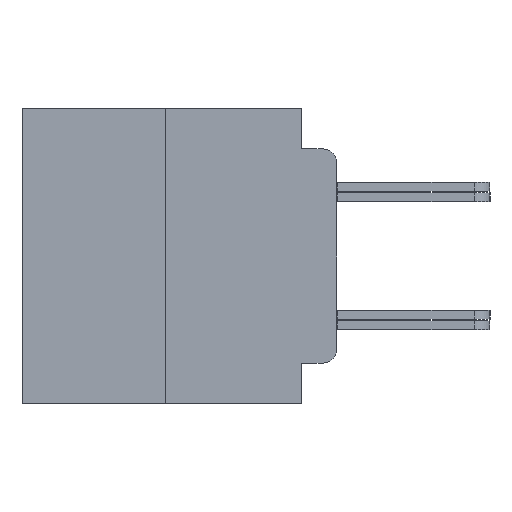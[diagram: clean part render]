
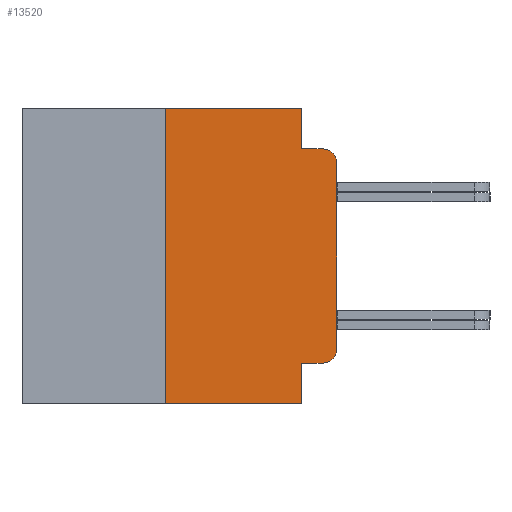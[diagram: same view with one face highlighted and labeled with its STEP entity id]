
A CAD part, left-side view. The second image highlights one B-rep face of the part: STEP entity #13520.
In plain terms, the highlighted planar face has unit normal (-1, 0, 0).
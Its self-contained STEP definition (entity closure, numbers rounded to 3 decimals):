
#203 = CARTESIAN_POINT ( 'NONE',  ( -75.603, 0.508, -3.975 ) ) ;
#330 = VECTOR ( 'NONE', #15667, 1000. ) ;
#479 = VERTEX_POINT ( 'NONE', #25853 ) ;
#786 = CARTESIAN_POINT ( 'NONE',  ( -75.603, 0.508, 3.467 ) ) ;
#1396 = LINE ( 'NONE', #4190, #27976 ) ;
#1812 = LINE ( 'NONE', #8970, #3211 ) ;
#2841 = CARTESIAN_POINT ( 'NONE',  ( -75.603, 0., -3.467 ) ) ;
#2872 = EDGE_CURVE ( 'NONE', #10562, #11289, #6207, .T. ) ;
#2905 = EDGE_CURVE ( 'NONE', #21259, #26325, #23056, .T. ) ;
#3078 = CARTESIAN_POINT ( 'NONE',  ( -75.603, 11.684, 5.486 ) ) ;
#3211 = VECTOR ( 'NONE', #4315, 1000. ) ;
#3571 = ORIENTED_EDGE ( 'NONE', *, *, #21143, .T. ) ;
#3697 = CARTESIAN_POINT ( 'NONE',  ( -75.603, 1.295, 0. ) ) ;
#3964 = VERTEX_POINT ( 'NONE', #2841 ) ;
#4078 = LINE ( 'NONE', #3697, #5091 ) ;
#4190 = CARTESIAN_POINT ( 'NONE',  ( -75.603, 0., 5.486 ) ) ;
#4315 = DIRECTION ( 'NONE',  ( 0., -1., 0. ) ) ;
#4521 = EDGE_CURVE ( 'NONE', #21259, #25367, #4078, .T. ) ;
#4785 = ORIENTED_EDGE ( 'NONE', *, *, #12134, .F. ) ;
#4992 = DIRECTION ( 'NONE',  ( 1., 0., 0. ) ) ;
#5076 = ORIENTED_EDGE ( 'NONE', *, *, #2905, .T. ) ;
#5091 = VECTOR ( 'NONE', #10548, 1000. ) ;
#5511 = DIRECTION ( 'NONE',  ( -1., 0., 0. ) ) ;
#6097 = CIRCLE ( 'NONE', #24256, 0.508 ) ;
#6207 = LINE ( 'NONE', #22207, #330 ) ;
#6872 = CARTESIAN_POINT ( 'NONE',  ( -75.603, 1.295, -3.975 ) ) ;
#6896 = EDGE_CURVE ( 'NONE', #479, #10562, #14738, .T. ) ;
#7248 = ORIENTED_EDGE ( 'NONE', *, *, #14729, .T. ) ;
#7509 = VERTEX_POINT ( 'NONE', #14539 ) ;
#7643 = DIRECTION ( 'NONE',  ( 0., 0., -1. ) ) ;
#8829 = ORIENTED_EDGE ( 'NONE', *, *, #27594, .F. ) ;
#8970 = CARTESIAN_POINT ( 'NONE',  ( -75.603, 1.295, 3.975 ) ) ;
#9094 = VERTEX_POINT ( 'NONE', #22954 ) ;
#9109 = VECTOR ( 'NONE', #11445, 1000. ) ;
#9337 = EDGE_CURVE ( 'NONE', #7509, #25367, #25652, .T. ) ;
#9553 = DIRECTION ( 'NONE',  ( 0., 0., -1. ) ) ;
#10394 = DIRECTION ( 'NONE',  ( -1., 0., 0. ) ) ;
#10522 = ORIENTED_EDGE ( 'NONE', *, *, #25203, .T. ) ;
#10548 = DIRECTION ( 'NONE',  ( 0., 0., -1. ) ) ;
#10562 = VERTEX_POINT ( 'NONE', #12122 ) ;
#11289 = VERTEX_POINT ( 'NONE', #14864 ) ;
#11445 = DIRECTION ( 'NONE',  ( 0., 0., 1. ) ) ;
#11871 = VECTOR ( 'NONE', #14793, 1000. ) ;
#12122 = CARTESIAN_POINT ( 'NONE',  ( -75.603, 1.295, 5.486 ) ) ;
#12134 = EDGE_CURVE ( 'NONE', #11289, #9094, #1812, .T. ) ;
#13520 = ADVANCED_FACE ( 'NONE', ( #25164 ), #20667, .F. ) ;
#13848 = CARTESIAN_POINT ( 'NONE',  ( -75.603, 1.295, -3.975 ) ) ;
#14024 = DIRECTION ( 'NONE',  ( 0., -1., 0. ) ) ;
#14539 = CARTESIAN_POINT ( 'NONE',  ( -75.603, 6.35, -5.486 ) ) ;
#14729 = EDGE_CURVE ( 'NONE', #24963, #9094, #16519, .T. ) ;
#14738 = LINE ( 'NONE', #27238, #24346 ) ;
#14746 = ORIENTED_EDGE ( 'NONE', *, *, #9337, .T. ) ;
#14793 = DIRECTION ( 'NONE',  ( 0., -1., 0. ) ) ;
#14864 = CARTESIAN_POINT ( 'NONE',  ( -75.603, 1.295, 3.975 ) ) ;
#15667 = DIRECTION ( 'NONE',  ( 0., 0., -1. ) ) ;
#16238 = ORIENTED_EDGE ( 'NONE', *, *, #4521, .F. ) ;
#16519 = CIRCLE ( 'NONE', #21732, 0.508 ) ;
#17395 = CARTESIAN_POINT ( 'NONE',  ( -75.603, 1.295, -5.486 ) ) ;
#19203 = CARTESIAN_POINT ( 'NONE',  ( -75.603, 11.684, -5.486 ) ) ;
#19952 = VECTOR ( 'NONE', #20852, 1000. ) ;
#19968 = CARTESIAN_POINT ( 'NONE',  ( -75.603, 6.35, -5.486 ) ) ;
#20146 = ORIENTED_EDGE ( 'NONE', *, *, #6896, .F. ) ;
#20667 = PLANE ( 'NONE',  #26903 ) ;
#20852 = DIRECTION ( 'NONE',  ( 0., -1., 0. ) ) ;
#21143 = EDGE_CURVE ( 'NONE', #3964, #24963, #1396, .T. ) ;
#21259 = VERTEX_POINT ( 'NONE', #6872 ) ;
#21732 = AXIS2_PLACEMENT_3D ( 'NONE', #786, #5511, #7643 ) ;
#22207 = CARTESIAN_POINT ( 'NONE',  ( -75.603, 1.295, 0. ) ) ;
#22954 = CARTESIAN_POINT ( 'NONE',  ( -75.603, 0.508, 3.975 ) ) ;
#23056 = LINE ( 'NONE', #13848, #19952 ) ;
#23532 = CARTESIAN_POINT ( 'NONE',  ( -75.603, 0.508, -3.467 ) ) ;
#24256 = AXIS2_PLACEMENT_3D ( 'NONE', #23532, #10394, #27936 ) ;
#24346 = VECTOR ( 'NONE', #14024, 1000. ) ;
#24963 = VERTEX_POINT ( 'NONE', #27350 ) ;
#25164 = FACE_OUTER_BOUND ( 'NONE', #27740, .T. ) ;
#25203 = EDGE_CURVE ( 'NONE', #26325, #3964, #6097, .T. ) ;
#25367 = VERTEX_POINT ( 'NONE', #17395 ) ;
#25652 = LINE ( 'NONE', #19203, #11871 ) ;
#25834 = ORIENTED_EDGE ( 'NONE', *, *, #2872, .F. ) ;
#25853 = CARTESIAN_POINT ( 'NONE',  ( -75.603, 6.35, 5.486 ) ) ;
#26325 = VERTEX_POINT ( 'NONE', #203 ) ;
#26903 = AXIS2_PLACEMENT_3D ( 'NONE', #3078, #4992, #9553 ) ;
#27238 = CARTESIAN_POINT ( 'NONE',  ( -75.603, 11.684, 5.486 ) ) ;
#27350 = CARTESIAN_POINT ( 'NONE',  ( -75.603, 0., 3.467 ) ) ;
#27366 = LINE ( 'NONE', #19968, #9109 ) ;
#27594 = EDGE_CURVE ( 'NONE', #7509, #479, #27366, .T. ) ;
#27740 = EDGE_LOOP ( 'NONE', ( #5076, #10522, #3571, #7248, #4785, #25834, #20146, #8829, #14746, #16238 ) ) ;
#27936 = DIRECTION ( 'NONE',  ( 0., 0., -1. ) ) ;
#27976 = VECTOR ( 'NONE', #28479, 1000. ) ;
#28479 = DIRECTION ( 'NONE',  ( 0., 0., 1. ) ) ;
